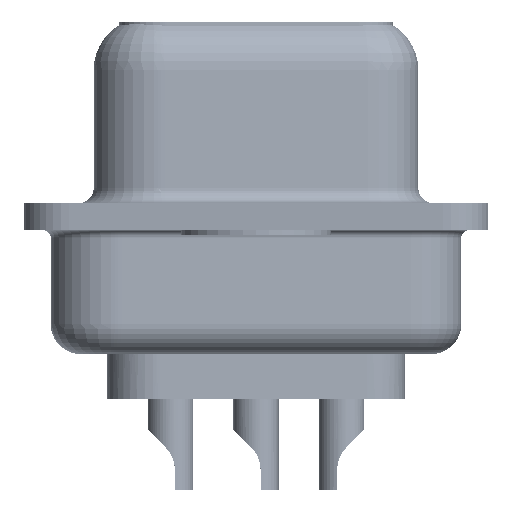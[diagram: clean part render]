
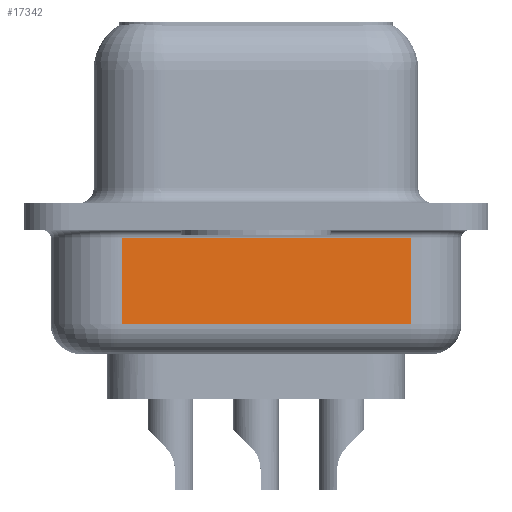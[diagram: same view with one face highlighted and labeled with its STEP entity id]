
A CAD part, left-side view. The second image highlights one B-rep face of the part: STEP entity #17342.
In plain terms, the highlighted planar face has unit normal (-0.985, -0.174, 0).
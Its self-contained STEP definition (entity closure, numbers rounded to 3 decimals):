
#584 = VERTEX_POINT ( 'NONE', #6038 ) ;
#1342 = VECTOR ( 'NONE', #23221, 1000. ) ;
#1410 = CARTESIAN_POINT ( 'NONE',  ( 2.93, 4.453, -4.55 ) ) ;
#2557 = LINE ( 'NONE', #19661, #32194 ) ;
#2646 = EDGE_CURVE ( 'NONE', #15317, #11775, #23000, .T. ) ;
#2752 = VECTOR ( 'NONE', #34339, 1000. ) ;
#3296 = CARTESIAN_POINT ( 'NONE',  ( 4.623, -5.147, -4.55 ) ) ;
#4367 = LINE ( 'NONE', #1410, #8857 ) ;
#4548 = DIRECTION ( 'NONE',  ( 0., 0., 1. ) ) ;
#6038 = CARTESIAN_POINT ( 'NONE',  ( 2.93, 4.453, -3.55 ) ) ;
#6131 = LINE ( 'NONE', #29332, #1342 ) ;
#8561 = EDGE_CURVE ( 'NONE', #11775, #27236, #2557, .T. ) ;
#8857 = VECTOR ( 'NONE', #4548, 1000. ) ;
#11775 = VERTEX_POINT ( 'NONE', #32747 ) ;
#11888 = CARTESIAN_POINT ( 'NONE',  ( 2.93, 4.453, -4.55 ) ) ;
#11928 = ORIENTED_EDGE ( 'NONE', *, *, #31955, .F. ) ;
#12196 = AXIS2_PLACEMENT_3D ( 'NONE', #11888, #17288, #23026 ) ;
#14870 = PLANE ( 'NONE',  #12196 ) ;
#15317 = VERTEX_POINT ( 'NONE', #36607 ) ;
#16372 = EDGE_LOOP ( 'NONE', ( #11928, #25781, #18653, #22338 ) ) ;
#17288 = DIRECTION ( 'NONE',  ( 0.985, 0.174, 0. ) ) ;
#17342 = ADVANCED_FACE ( 'NONE', ( #20241 ), #14870, .F. ) ;
#18653 = ORIENTED_EDGE ( 'NONE', *, *, #2646, .T. ) ;
#19661 = CARTESIAN_POINT ( 'NONE',  ( 2.93, 4.453, -0.7 ) ) ;
#20241 = FACE_OUTER_BOUND ( 'NONE', #16372, .T. ) ;
#22338 = ORIENTED_EDGE ( 'NONE', *, *, #8561, .T. ) ;
#23000 = LINE ( 'NONE', #3296, #2752 ) ;
#23026 = DIRECTION ( 'NONE',  ( -0.174, 0.985, 0. ) ) ;
#23221 = DIRECTION ( 'NONE',  ( 0.174, -0.985, 0. ) ) ;
#25781 = ORIENTED_EDGE ( 'NONE', *, *, #36339, .T. ) ;
#27236 = VERTEX_POINT ( 'NONE', #32705 ) ;
#28541 = DIRECTION ( 'NONE',  ( -0.174, 0.985, 0. ) ) ;
#29332 = CARTESIAN_POINT ( 'NONE',  ( 2.93, 4.453, -3.55 ) ) ;
#31955 = EDGE_CURVE ( 'NONE', #584, #27236, #4367, .T. ) ;
#32194 = VECTOR ( 'NONE', #28541, 1000. ) ;
#32705 = CARTESIAN_POINT ( 'NONE',  ( 2.93, 4.453, -0.7 ) ) ;
#32747 = CARTESIAN_POINT ( 'NONE',  ( 4.623, -5.147, -0.7 ) ) ;
#34339 = DIRECTION ( 'NONE',  ( 0., 0., 1. ) ) ;
#36339 = EDGE_CURVE ( 'NONE', #584, #15317, #6131, .T. ) ;
#36607 = CARTESIAN_POINT ( 'NONE',  ( 4.623, -5.147, -3.55 ) ) ;
